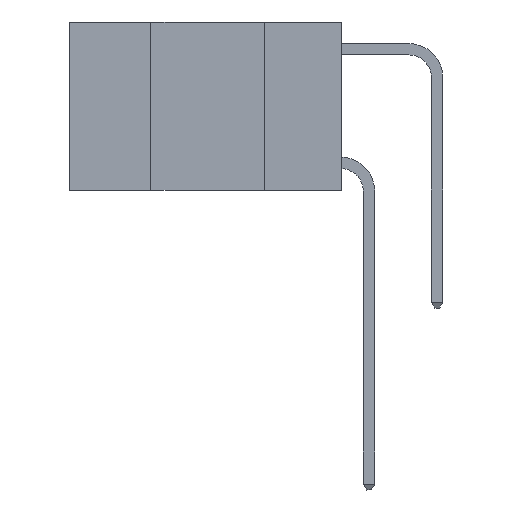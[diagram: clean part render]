
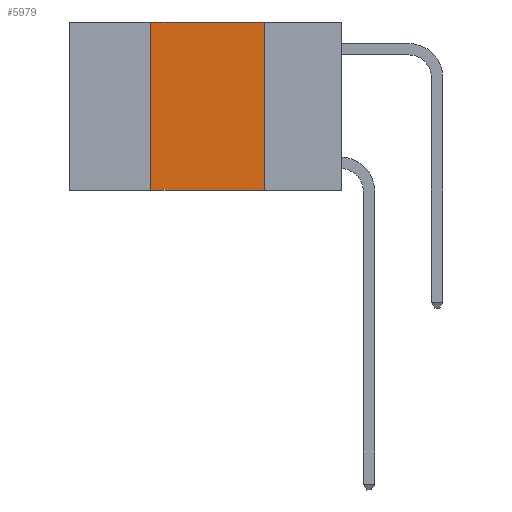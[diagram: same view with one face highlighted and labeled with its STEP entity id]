
A CAD part, left-side view. The second image highlights one B-rep face of the part: STEP entity #5979.
In plain terms, the highlighted planar face has unit normal (-1, 0, 0).
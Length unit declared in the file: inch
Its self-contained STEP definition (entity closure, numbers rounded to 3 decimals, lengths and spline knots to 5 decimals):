
#766 = VERTEX_POINT ( 'NONE', #7826 ) ;
#1205 = EDGE_CURVE ( 'NONE', #3736, #1295, #10638, .T. ) ;
#1232 = AXIS2_PLACEMENT_3D ( 'NONE', #11156, #5816, #6634 ) ;
#1295 = VERTEX_POINT ( 'NONE', #2810 ) ;
#1543 = DIRECTION ( 'NONE',  ( 0., 0., 1. ) ) ;
#1582 = CARTESIAN_POINT ( 'NONE',  ( 0., 0.42, -0.37 ) ) ;
#1776 = ORIENTED_EDGE ( 'NONE', *, *, #1982, .F. ) ;
#1982 = EDGE_CURVE ( 'NONE', #766, #3736, #8972, .T. ) ;
#2565 = DIRECTION ( 'NONE',  ( 0., 0., -1. ) ) ;
#2623 = LINE ( 'NONE', #6215, #6393 ) ;
#2810 = CARTESIAN_POINT ( 'NONE',  ( 0., 0.17, -0.37 ) ) ;
#3449 = ORIENTED_EDGE ( 'NONE', *, *, #8268, .F. ) ;
#3563 = VECTOR ( 'NONE', #5270, 39.37008 ) ;
#3736 = VERTEX_POINT ( 'NONE', #5099 ) ;
#5099 = CARTESIAN_POINT ( 'NONE',  ( 0., 0.17, 0. ) ) ;
#5270 = DIRECTION ( 'NONE',  ( 0., -1., 0. ) ) ;
#5816 = DIRECTION ( 'NONE',  ( 1., 0., 0. ) ) ;
#5979 = ADVANCED_FACE ( 'NONE', ( #7573 ), #10345, .F. ) ;
#6215 = CARTESIAN_POINT ( 'NONE',  ( 0., 0.6, -0.37 ) ) ;
#6393 = VECTOR ( 'NONE', #8822, 39.37008 ) ;
#6634 = DIRECTION ( 'NONE',  ( 0., 0., -1. ) ) ;
#6646 = ORIENTED_EDGE ( 'NONE', *, *, #9197, .T. ) ;
#6719 = LINE ( 'NONE', #6788, #8796 ) ;
#6788 = CARTESIAN_POINT ( 'NONE',  ( 0., 0.42, 0. ) ) ;
#7024 = CARTESIAN_POINT ( 'NONE',  ( 0., 0.6, 0. ) ) ;
#7169 = CARTESIAN_POINT ( 'NONE',  ( 0., 0.17, 0. ) ) ;
#7471 = VERTEX_POINT ( 'NONE', #1582 ) ;
#7573 = FACE_OUTER_BOUND ( 'NONE', #8421, .T. ) ;
#7826 = CARTESIAN_POINT ( 'NONE',  ( 0., 0.42, 0. ) ) ;
#8268 = EDGE_CURVE ( 'NONE', #7471, #766, #6719, .T. ) ;
#8421 = EDGE_LOOP ( 'NONE', ( #10627, #1776, #3449, #6646 ) ) ;
#8447 = VECTOR ( 'NONE', #2565, 39.37008 ) ;
#8796 = VECTOR ( 'NONE', #1543, 39.37008 ) ;
#8822 = DIRECTION ( 'NONE',  ( 0., -1., 0. ) ) ;
#8972 = LINE ( 'NONE', #7024, #3563 ) ;
#9197 = EDGE_CURVE ( 'NONE', #7471, #1295, #2623, .T. ) ;
#10345 = PLANE ( 'NONE',  #1232 ) ;
#10627 = ORIENTED_EDGE ( 'NONE', *, *, #1205, .F. ) ;
#10638 = LINE ( 'NONE', #7169, #8447 ) ;
#11156 = CARTESIAN_POINT ( 'NONE',  ( 0., 0.6, 0. ) ) ;
